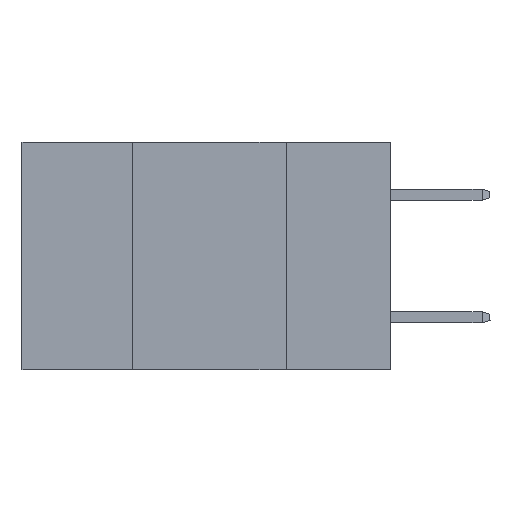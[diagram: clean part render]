
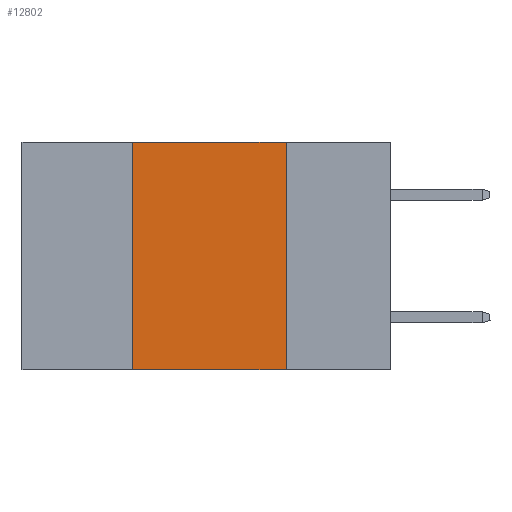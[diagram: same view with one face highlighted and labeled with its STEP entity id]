
A CAD part, left-side view. The second image highlights one B-rep face of the part: STEP entity #12802.
In plain terms, the highlighted planar face has unit normal (-1, 0, 0).
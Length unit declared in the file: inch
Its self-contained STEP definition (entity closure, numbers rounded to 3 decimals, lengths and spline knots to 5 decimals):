
#95 = ORIENTED_EDGE ( 'NONE', *, *, #2930, .F. ) ;
#603 = VECTOR ( 'NONE', #11259, 39.37008 ) ;
#643 = VECTOR ( 'NONE', #2830, 39.37008 ) ;
#826 = ORIENTED_EDGE ( 'NONE', *, *, #5274, .F. ) ;
#1195 = PLANE ( 'NONE',  #3412 ) ;
#1818 = ORIENTED_EDGE ( 'NONE', *, *, #6233, .F. ) ;
#1912 = CARTESIAN_POINT ( 'NONE',  ( 0., 0.6, 0. ) ) ;
#2049 = CARTESIAN_POINT ( 'NONE',  ( 0., 0.42, 0. ) ) ;
#2648 = EDGE_CURVE ( 'NONE', #11139, #9654, #7892, .T. ) ;
#2830 = DIRECTION ( 'NONE',  ( 0., 0., 1. ) ) ;
#2930 = EDGE_CURVE ( 'NONE', #9318, #11590, #7591, .T. ) ;
#3141 = CARTESIAN_POINT ( 'NONE',  ( 0., 0.42, 0. ) ) ;
#3412 = AXIS2_PLACEMENT_3D ( 'NONE', #5487, #10457, #4506 ) ;
#3592 = LINE ( 'NONE', #2049, #643 ) ;
#3790 = DIRECTION ( 'NONE',  ( 0., -1., 0. ) ) ;
#4485 = VECTOR ( 'NONE', #10927, 39.37008 ) ;
#4506 = DIRECTION ( 'NONE',  ( 0., 0., -1. ) ) ;
#4541 = EDGE_LOOP ( 'NONE', ( #1818, #95, #826, #9183 ) ) ;
#4758 = CARTESIAN_POINT ( 'NONE',  ( 0., 0.17, 0. ) ) ;
#5274 = EDGE_CURVE ( 'NONE', #11139, #9318, #3592, .T. ) ;
#5487 = CARTESIAN_POINT ( 'NONE',  ( 0., 0.6, 0. ) ) ;
#6132 = CARTESIAN_POINT ( 'NONE',  ( 0., 0.42, -0.37 ) ) ;
#6151 = CARTESIAN_POINT ( 'NONE',  ( 0., 0.6, -0.37 ) ) ;
#6233 = EDGE_CURVE ( 'NONE', #11590, #9654, #9010, .T. ) ;
#7591 = LINE ( 'NONE', #1912, #9555 ) ;
#7892 = LINE ( 'NONE', #6151, #4485 ) ;
#9010 = LINE ( 'NONE', #11572, #603 ) ;
#9183 = ORIENTED_EDGE ( 'NONE', *, *, #2648, .T. ) ;
#9318 = VERTEX_POINT ( 'NONE', #3141 ) ;
#9555 = VECTOR ( 'NONE', #3790, 39.37008 ) ;
#9654 = VERTEX_POINT ( 'NONE', #10774 ) ;
#10457 = DIRECTION ( 'NONE',  ( 1., 0., 0. ) ) ;
#10759 = FACE_OUTER_BOUND ( 'NONE', #4541, .T. ) ;
#10774 = CARTESIAN_POINT ( 'NONE',  ( 0., 0.17, -0.37 ) ) ;
#10927 = DIRECTION ( 'NONE',  ( 0., -1., 0. ) ) ;
#11139 = VERTEX_POINT ( 'NONE', #6132 ) ;
#11259 = DIRECTION ( 'NONE',  ( 0., 0., -1. ) ) ;
#11572 = CARTESIAN_POINT ( 'NONE',  ( 0., 0.17, 0. ) ) ;
#11590 = VERTEX_POINT ( 'NONE', #4758 ) ;
#12802 = ADVANCED_FACE ( 'NONE', ( #10759 ), #1195, .F. ) ;
